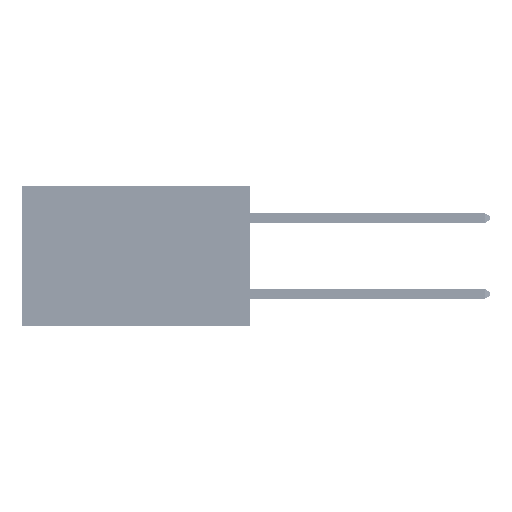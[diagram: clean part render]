
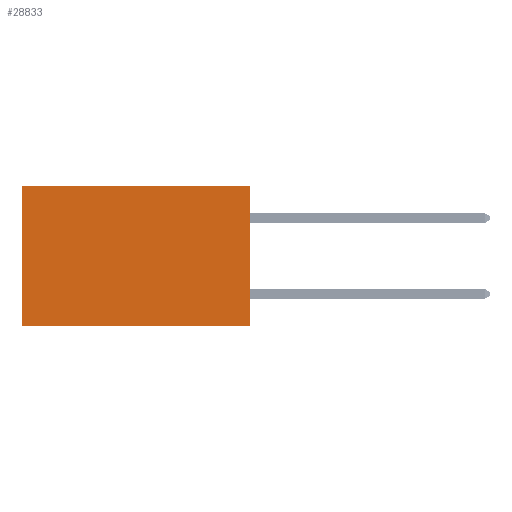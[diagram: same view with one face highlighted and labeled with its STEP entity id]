
A CAD part, left-side view. The second image highlights one B-rep face of the part: STEP entity #28833.
In plain terms, the highlighted planar face has unit normal (-1, 0, 0).
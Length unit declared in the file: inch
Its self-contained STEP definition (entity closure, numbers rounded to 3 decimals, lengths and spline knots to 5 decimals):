
#46 = CARTESIAN_POINT ( 'NONE',  ( 0.2875, 0., 0. ) ) ;
#1424 = CARTESIAN_POINT ( 'NONE',  ( 0.2875, 0.6, 0. ) ) ;
#1936 = LINE ( 'NONE', #46, #39999 ) ;
#2569 = AXIS2_PLACEMENT_3D ( 'NONE', #39346, #43302, #39182 ) ;
#2621 = CARTESIAN_POINT ( 'NONE',  ( 0.2875, 0., 0. ) ) ;
#3445 = VECTOR ( 'NONE', #29421, 39.37008 ) ;
#3473 = PLANE ( 'NONE',  #2569 ) ;
#4587 = VERTEX_POINT ( 'NONE', #45538 ) ;
#5396 = VERTEX_POINT ( 'NONE', #34298 ) ;
#5688 = ORIENTED_EDGE ( 'NONE', *, *, #27595, .F. ) ;
#7087 = LINE ( 'NONE', #35555, #13851 ) ;
#7125 = CARTESIAN_POINT ( 'NONE',  ( 0.2875, 0.6, 0. ) ) ;
#8242 = DIRECTION ( 'NONE',  ( 0., 1., 0. ) ) ;
#8829 = VERTEX_POINT ( 'NONE', #48667 ) ;
#10762 = EDGE_LOOP ( 'NONE', ( #29098, #5688, #17259, #16915 ) ) ;
#13743 = FACE_OUTER_BOUND ( 'NONE', #10762, .T. ) ;
#13851 = VECTOR ( 'NONE', #8242, 39.37008 ) ;
#13901 = LINE ( 'NONE', #2621, #3445 ) ;
#16915 = ORIENTED_EDGE ( 'NONE', *, *, #27268, .T. ) ;
#17010 = VERTEX_POINT ( 'NONE', #7125 ) ;
#17259 = ORIENTED_EDGE ( 'NONE', *, *, #24515, .F. ) ;
#22436 = VECTOR ( 'NONE', #44525, 39.37008 ) ;
#24515 = EDGE_CURVE ( 'NONE', #4587, #5396, #1936, .T. ) ;
#26722 = LINE ( 'NONE', #1424, #22436 ) ;
#27268 = EDGE_CURVE ( 'NONE', #4587, #17010, #13901, .T. ) ;
#27595 = EDGE_CURVE ( 'NONE', #5396, #8829, #7087, .T. ) ;
#28833 = ADVANCED_FACE ( 'NONE', ( #13743 ), #3473, .F. ) ;
#29098 = ORIENTED_EDGE ( 'NONE', *, *, #34355, .T. ) ;
#29421 = DIRECTION ( 'NONE',  ( 0., 1., 0. ) ) ;
#31002 = DIRECTION ( 'NONE',  ( 0., 0., -1. ) ) ;
#34298 = CARTESIAN_POINT ( 'NONE',  ( 0.2875, 0., -0.37 ) ) ;
#34355 = EDGE_CURVE ( 'NONE', #17010, #8829, #26722, .T. ) ;
#35555 = CARTESIAN_POINT ( 'NONE',  ( 0.2875, 0., -0.37 ) ) ;
#39182 = DIRECTION ( 'NONE',  ( 0., 0., -1. ) ) ;
#39346 = CARTESIAN_POINT ( 'NONE',  ( 0.2875, 0., 0. ) ) ;
#39999 = VECTOR ( 'NONE', #31002, 39.37008 ) ;
#43302 = DIRECTION ( 'NONE',  ( 1., 0., 0. ) ) ;
#44525 = DIRECTION ( 'NONE',  ( 0., 0., -1. ) ) ;
#45538 = CARTESIAN_POINT ( 'NONE',  ( 0.2875, 0., 0. ) ) ;
#48667 = CARTESIAN_POINT ( 'NONE',  ( 0.2875, 0.6, -0.37 ) ) ;
